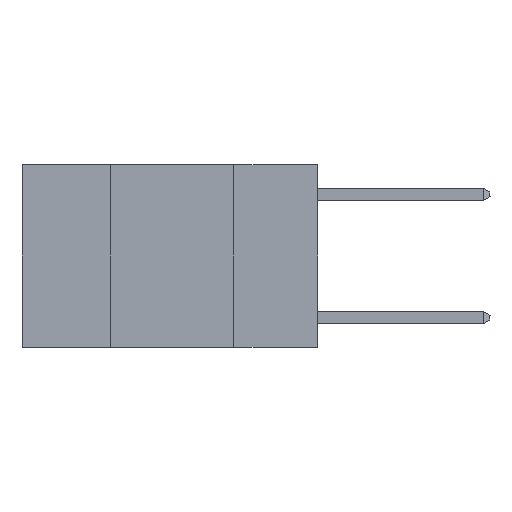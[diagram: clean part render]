
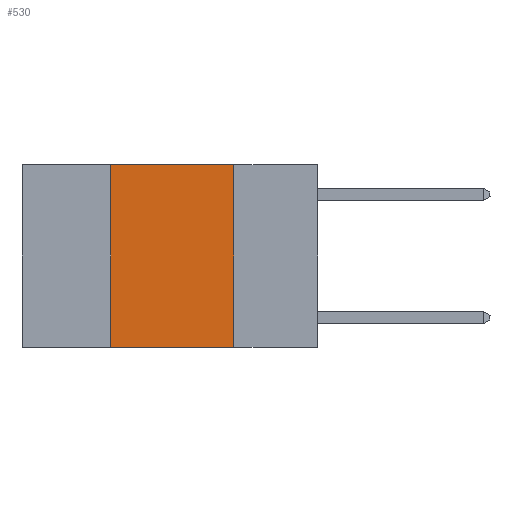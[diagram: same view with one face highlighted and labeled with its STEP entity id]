
A CAD part, left-side view. The second image highlights one B-rep face of the part: STEP entity #530.
In plain terms, the highlighted planar face has unit normal (-1, 0, 0).
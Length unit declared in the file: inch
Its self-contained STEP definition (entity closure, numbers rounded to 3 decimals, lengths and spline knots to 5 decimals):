
#530 = ADVANCED_FACE ( 'NONE', ( #26829 ), #17870, .F. ) ;
#1210 = CARTESIAN_POINT ( 'NONE',  ( 0., 0.6, 0. ) ) ;
#1733 = CARTESIAN_POINT ( 'NONE',  ( 0., 0.17, 0. ) ) ;
#2228 = CARTESIAN_POINT ( 'NONE',  ( 0., 0.42, 0. ) ) ;
#4027 = EDGE_CURVE ( 'NONE', #23590, #12855, #6302, .T. ) ;
#5015 = VECTOR ( 'NONE', #7501, 39.37008 ) ;
#6302 = LINE ( 'NONE', #6589, #12356 ) ;
#6589 = CARTESIAN_POINT ( 'NONE',  ( 0., 0.42, 0. ) ) ;
#7501 = DIRECTION ( 'NONE',  ( 0., -1., 0. ) ) ;
#7586 = VERTEX_POINT ( 'NONE', #16316 ) ;
#8332 = VERTEX_POINT ( 'NONE', #23790 ) ;
#12356 = VECTOR ( 'NONE', #14988, 39.37008 ) ;
#12435 = AXIS2_PLACEMENT_3D ( 'NONE', #26268, #13315, #26543 ) ;
#12855 = VERTEX_POINT ( 'NONE', #2228 ) ;
#12987 = LINE ( 'NONE', #1733, #15077 ) ;
#13315 = DIRECTION ( 'NONE',  ( 1., 0., 0. ) ) ;
#13778 = ORIENTED_EDGE ( 'NONE', *, *, #18836, .T. ) ;
#14608 = ORIENTED_EDGE ( 'NONE', *, *, #17233, .F. ) ;
#14988 = DIRECTION ( 'NONE',  ( 0., 0., 1. ) ) ;
#15077 = VECTOR ( 'NONE', #25785, 39.37008 ) ;
#16316 = CARTESIAN_POINT ( 'NONE',  ( 0., 0.17, 0. ) ) ;
#16749 = ORIENTED_EDGE ( 'NONE', *, *, #4027, .F. ) ;
#17233 = EDGE_CURVE ( 'NONE', #7586, #8332, #12987, .T. ) ;
#17870 = PLANE ( 'NONE',  #12435 ) ;
#18452 = EDGE_CURVE ( 'NONE', #12855, #7586, #26846, .T. ) ;
#18529 = CARTESIAN_POINT ( 'NONE',  ( 0., 0.6, -0.37 ) ) ;
#18836 = EDGE_CURVE ( 'NONE', #23590, #8332, #27062, .T. ) ;
#22149 = ORIENTED_EDGE ( 'NONE', *, *, #18452, .F. ) ;
#22781 = DIRECTION ( 'NONE',  ( 0., -1., 0. ) ) ;
#23590 = VERTEX_POINT ( 'NONE', #24028 ) ;
#23790 = CARTESIAN_POINT ( 'NONE',  ( 0., 0.17, -0.37 ) ) ;
#24028 = CARTESIAN_POINT ( 'NONE',  ( 0., 0.42, -0.37 ) ) ;
#25017 = VECTOR ( 'NONE', #22781, 39.37008 ) ;
#25785 = DIRECTION ( 'NONE',  ( 0., 0., -1. ) ) ;
#26268 = CARTESIAN_POINT ( 'NONE',  ( 0., 0.6, 0. ) ) ;
#26543 = DIRECTION ( 'NONE',  ( 0., 0., -1. ) ) ;
#26829 = FACE_OUTER_BOUND ( 'NONE', #27179, .T. ) ;
#26846 = LINE ( 'NONE', #1210, #5015 ) ;
#27062 = LINE ( 'NONE', #18529, #25017 ) ;
#27179 = EDGE_LOOP ( 'NONE', ( #14608, #22149, #16749, #13778 ) ) ;
